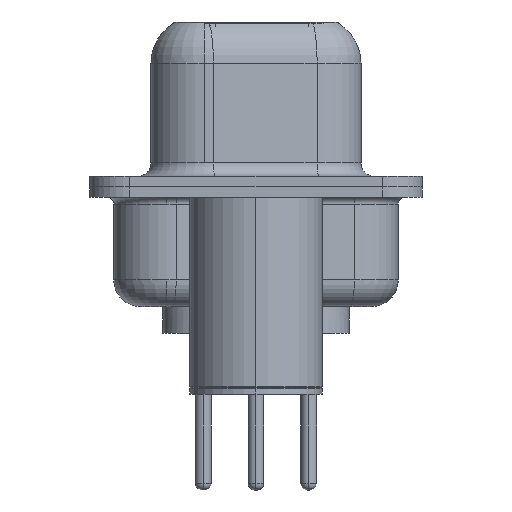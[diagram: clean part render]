
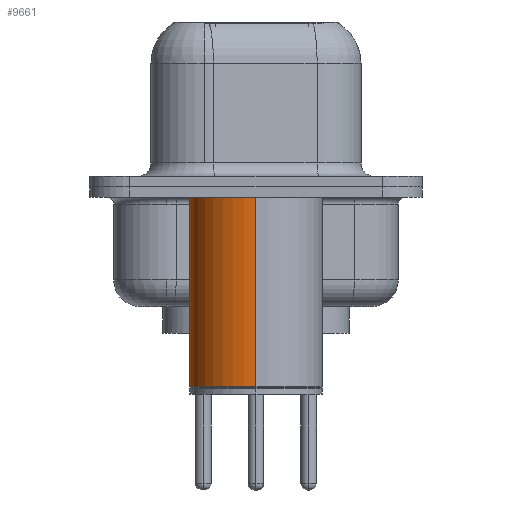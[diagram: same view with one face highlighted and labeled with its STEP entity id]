
A CAD part, left-side view. The second image highlights one B-rep face of the part: STEP entity #9661.
In plain terms, the highlighted cylindrical face has radius 2.5 mm (diameter 5 mm), a partial arc.
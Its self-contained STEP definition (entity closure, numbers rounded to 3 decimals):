
#1575 = VECTOR ( 'NONE', #13604, 1000. ) ;
#1687 = CARTESIAN_POINT ( 'NONE',  ( 0., 0., -0.4 ) ) ;
#1739 = DIRECTION ( 'NONE',  ( 0., 0., 1. ) ) ;
#2002 = CARTESIAN_POINT ( 'NONE',  ( -2.5, 0., -0.4 ) ) ;
#2157 = VECTOR ( 'NONE', #19567, 1000. ) ;
#2805 = ORIENTED_EDGE ( 'NONE', *, *, #15218, .F. ) ;
#3512 = CYLINDRICAL_SURFACE ( 'NONE', #13083, 2.5 ) ;
#3710 = DIRECTION ( 'NONE',  ( 1., 0., 0. ) ) ;
#4367 = ORIENTED_EDGE ( 'NONE', *, *, #13664, .T. ) ;
#4702 = CARTESIAN_POINT ( 'NONE',  ( 2.5, 0., 0.581 ) ) ;
#4744 = VERTEX_POINT ( 'NONE', #8858 ) ;
#5489 = DIRECTION ( 'NONE',  ( 0., 0., 1. ) ) ;
#6410 = VERTEX_POINT ( 'NONE', #8253 ) ;
#7972 = CARTESIAN_POINT ( 'NONE',  ( -2.5, 0., 0.581 ) ) ;
#8253 = CARTESIAN_POINT ( 'NONE',  ( -2.5, 0., -7.525 ) ) ;
#8610 = CIRCLE ( 'NONE', #21101, 2.5 ) ;
#8809 = EDGE_CURVE ( 'NONE', #8861, #6410, #8610, .T. ) ;
#8858 = CARTESIAN_POINT ( 'NONE',  ( 2.5, 0., -0.4 ) ) ;
#8861 = VERTEX_POINT ( 'NONE', #15044 ) ;
#9661 = ADVANCED_FACE ( 'NONE', ( #12297 ), #3512, .T. ) ;
#9797 = LINE ( 'NONE', #7972, #1575 ) ;
#10465 = DIRECTION ( 'NONE',  ( 0., 0., 1. ) ) ;
#10996 = CARTESIAN_POINT ( 'NONE',  ( 0., 0., -7.525 ) ) ;
#12297 = FACE_OUTER_BOUND ( 'NONE', #12408, .T. ) ;
#12408 = EDGE_LOOP ( 'NONE', ( #16679, #4367, #12646, #2805 ) ) ;
#12646 = ORIENTED_EDGE ( 'NONE', *, *, #21224, .F. ) ;
#12659 = AXIS2_PLACEMENT_3D ( 'NONE', #1687, #5489, #20362 ) ;
#12879 = DIRECTION ( 'NONE',  ( 1., 0., 0. ) ) ;
#13083 = AXIS2_PLACEMENT_3D ( 'NONE', #15852, #10465, #12879 ) ;
#13604 = DIRECTION ( 'NONE',  ( 0., 0., 1. ) ) ;
#13664 = EDGE_CURVE ( 'NONE', #6410, #22204, #9797, .T. ) ;
#14198 = LINE ( 'NONE', #4702, #2157 ) ;
#15044 = CARTESIAN_POINT ( 'NONE',  ( 2.5, 0., -7.525 ) ) ;
#15218 = EDGE_CURVE ( 'NONE', #8861, #4744, #14198, .T. ) ;
#15852 = CARTESIAN_POINT ( 'NONE',  ( 0., 0., 0.581 ) ) ;
#16679 = ORIENTED_EDGE ( 'NONE', *, *, #8809, .T. ) ;
#19567 = DIRECTION ( 'NONE',  ( 0., 0., 1. ) ) ;
#20362 = DIRECTION ( 'NONE',  ( 1., 0., 0. ) ) ;
#21101 = AXIS2_PLACEMENT_3D ( 'NONE', #10996, #1739, #3710 ) ;
#21224 = EDGE_CURVE ( 'NONE', #4744, #22204, #24013, .T. ) ;
#22204 = VERTEX_POINT ( 'NONE', #2002 ) ;
#24013 = CIRCLE ( 'NONE', #12659, 2.5 ) ;
